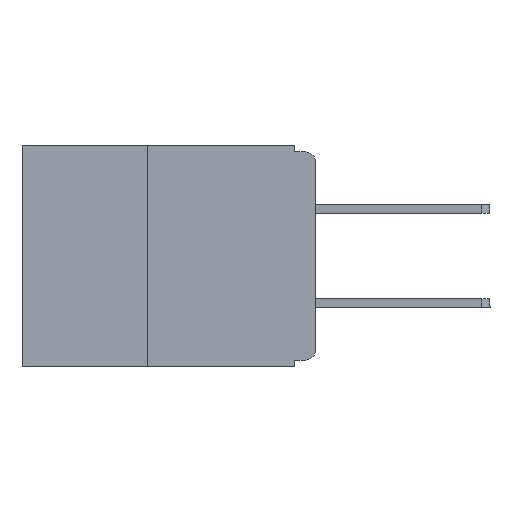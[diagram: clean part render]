
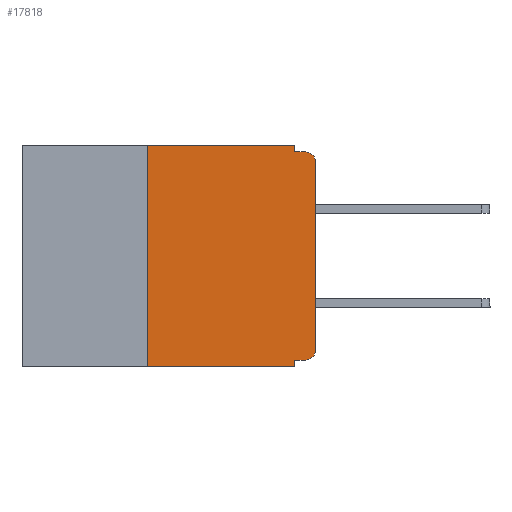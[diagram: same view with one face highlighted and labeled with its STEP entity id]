
A CAD part, left-side view. The second image highlights one B-rep face of the part: STEP entity #17818.
In plain terms, the highlighted planar face has unit normal (-1, 0, 0).
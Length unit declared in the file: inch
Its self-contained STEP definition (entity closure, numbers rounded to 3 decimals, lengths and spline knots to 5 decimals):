
#8 = CARTESIAN_POINT ( 'NONE',  ( 0., 0., 0. ) ) ;
#194 = CARTESIAN_POINT ( 'NONE',  ( 0., 0.25, 0. ) ) ;
#437 = LINE ( 'NONE', #5873, #7872 ) ;
#478 = DIRECTION ( 'NONE',  ( 0., 0., -1. ) ) ;
#487 = EDGE_CURVE ( 'NONE', #11605, #11095, #6424, .T. ) ;
#613 = ORIENTED_EDGE ( 'NONE', *, *, #2300, .F. ) ;
#980 = ORIENTED_EDGE ( 'NONE', *, *, #11216, .F. ) ;
#1407 = VERTEX_POINT ( 'NONE', #10038 ) ;
#1520 = DIRECTION ( 'NONE',  ( 0., 0., -1. ) ) ;
#1731 = LINE ( 'NONE', #17269, #12561 ) ;
#2257 = VECTOR ( 'NONE', #6563, 39.37008 ) ;
#2291 = AXIS2_PLACEMENT_3D ( 'NONE', #16004, #10372, #1520 ) ;
#2300 = EDGE_CURVE ( 'NONE', #6017, #14107, #12139, .T. ) ;
#2339 = ORIENTED_EDGE ( 'NONE', *, *, #15808, .F. ) ;
#2423 = VECTOR ( 'NONE', #478, 39.37008 ) ;
#2512 = CARTESIAN_POINT ( 'NONE',  ( 0., 0.015, -0.32 ) ) ;
#2629 = CARTESIAN_POINT ( 'NONE',  ( 0., 0.437, -0.33 ) ) ;
#2666 = EDGE_CURVE ( 'NONE', #6945, #1407, #1731, .T. ) ;
#2817 = VERTEX_POINT ( 'NONE', #13098 ) ;
#2829 = DIRECTION ( 'NONE',  ( 0., 0., -1. ) ) ;
#2949 = ORIENTED_EDGE ( 'NONE', *, *, #8596, .T. ) ;
#3160 = CARTESIAN_POINT ( 'NONE',  ( 0., 0.031, -0.33 ) ) ;
#3184 = EDGE_CURVE ( 'NONE', #6945, #11605, #4705, .T. ) ;
#3219 = LINE ( 'NONE', #2629, #10596 ) ;
#3246 = CARTESIAN_POINT ( 'NONE',  ( 0., 0.015, -0.025 ) ) ;
#3524 = VERTEX_POINT ( 'NONE', #194 ) ;
#4104 = DIRECTION ( 'NONE',  ( 0., -1., 0. ) ) ;
#4276 = EDGE_CURVE ( 'NONE', #3524, #2817, #437, .T. ) ;
#4498 = ORIENTED_EDGE ( 'NONE', *, *, #487, .T. ) ;
#4705 = CIRCLE ( 'NONE', #18412, 0.015 ) ;
#4715 = DIRECTION ( 'NONE',  ( 0., 0., -1. ) ) ;
#5078 = CARTESIAN_POINT ( 'NONE',  ( 0., 0.25, -0.33 ) ) ;
#5379 = ORIENTED_EDGE ( 'NONE', *, *, #3184, .T. ) ;
#5850 = DIRECTION ( 'NONE',  ( 0., -1., 0. ) ) ;
#5873 = CARTESIAN_POINT ( 'NONE',  ( 0., 0.437, 0. ) ) ;
#6017 = VERTEX_POINT ( 'NONE', #13529 ) ;
#6424 = LINE ( 'NONE', #8, #17345 ) ;
#6521 = FACE_OUTER_BOUND ( 'NONE', #8754, .T. ) ;
#6563 = DIRECTION ( 'NONE',  ( 0., 0., 1. ) ) ;
#6603 = VERTEX_POINT ( 'NONE', #3160 ) ;
#6945 = VERTEX_POINT ( 'NONE', #2512 ) ;
#7561 = CARTESIAN_POINT ( 'NONE',  ( 0., 0., -0.025 ) ) ;
#7872 = VECTOR ( 'NONE', #5850, 39.37008 ) ;
#8501 = ORIENTED_EDGE ( 'NONE', *, *, #14318, .F. ) ;
#8596 = EDGE_CURVE ( 'NONE', #11583, #6603, #3219, .T. ) ;
#8754 = EDGE_LOOP ( 'NONE', ( #4498, #16164, #613, #980, #10510, #2339, #2949, #8501, #18348, #5379 ) ) ;
#8821 = CARTESIAN_POINT ( 'NONE',  ( 0., 0., -0.305 ) ) ;
#8910 = EDGE_CURVE ( 'NONE', #11095, #14107, #16938, .T. ) ;
#9555 = CARTESIAN_POINT ( 'NONE',  ( 0., 0.015, -0.01 ) ) ;
#9629 = VECTOR ( 'NONE', #2829, 39.37008 ) ;
#10038 = CARTESIAN_POINT ( 'NONE',  ( 0., 0.031, -0.32 ) ) ;
#10268 = CARTESIAN_POINT ( 'NONE',  ( 0., 0.25, -0.33 ) ) ;
#10372 = DIRECTION ( 'NONE',  ( 1., 0., 0. ) ) ;
#10510 = ORIENTED_EDGE ( 'NONE', *, *, #4276, .F. ) ;
#10596 = VECTOR ( 'NONE', #4104, 39.37008 ) ;
#11095 = VERTEX_POINT ( 'NONE', #7561 ) ;
#11216 = EDGE_CURVE ( 'NONE', #2817, #6017, #14070, .T. ) ;
#11583 = VERTEX_POINT ( 'NONE', #10268 ) ;
#11605 = VERTEX_POINT ( 'NONE', #8821 ) ;
#11612 = AXIS2_PLACEMENT_3D ( 'NONE', #3246, #13475, #4715 ) ;
#11639 = DIRECTION ( 'NONE',  ( 0., 0., -1. ) ) ;
#11665 = CARTESIAN_POINT ( 'NONE',  ( 0., 0.031, -0.33 ) ) ;
#11726 = CARTESIAN_POINT ( 'NONE',  ( 0., 0.015, -0.305 ) ) ;
#11880 = DIRECTION ( 'NONE',  ( 0., -1., 0. ) ) ;
#11913 = DIRECTION ( 'NONE',  ( -1., 0., 0. ) ) ;
#12139 = LINE ( 'NONE', #13084, #16666 ) ;
#12561 = VECTOR ( 'NONE', #14027, 39.37008 ) ;
#13034 = LINE ( 'NONE', #5078, #2257 ) ;
#13084 = CARTESIAN_POINT ( 'NONE',  ( 0., 0., -0.01 ) ) ;
#13098 = CARTESIAN_POINT ( 'NONE',  ( 0., 0.031, 0. ) ) ;
#13475 = DIRECTION ( 'NONE',  ( -1., 0., 0. ) ) ;
#13529 = CARTESIAN_POINT ( 'NONE',  ( 0., 0.031, -0.01 ) ) ;
#14027 = DIRECTION ( 'NONE',  ( 0., 1., 0. ) ) ;
#14070 = LINE ( 'NONE', #17769, #2423 ) ;
#14107 = VERTEX_POINT ( 'NONE', #9555 ) ;
#14318 = EDGE_CURVE ( 'NONE', #1407, #6603, #16294, .T. ) ;
#14752 = DIRECTION ( 'NONE',  ( 0., 0., 1. ) ) ;
#15808 = EDGE_CURVE ( 'NONE', #11583, #3524, #13034, .T. ) ;
#16004 = CARTESIAN_POINT ( 'NONE',  ( 0., 0.437, 0. ) ) ;
#16164 = ORIENTED_EDGE ( 'NONE', *, *, #8910, .T. ) ;
#16294 = LINE ( 'NONE', #11665, #9629 ) ;
#16666 = VECTOR ( 'NONE', #11880, 39.37008 ) ;
#16938 = CIRCLE ( 'NONE', #11612, 0.015 ) ;
#17269 = CARTESIAN_POINT ( 'NONE',  ( 0., 0., -0.32 ) ) ;
#17345 = VECTOR ( 'NONE', #14752, 39.37008 ) ;
#17769 = CARTESIAN_POINT ( 'NONE',  ( 0., 0.031, 0. ) ) ;
#17818 = ADVANCED_FACE ( 'NONE', ( #6521 ), #18645, .F. ) ;
#18348 = ORIENTED_EDGE ( 'NONE', *, *, #2666, .F. ) ;
#18412 = AXIS2_PLACEMENT_3D ( 'NONE', #11726, #11913, #11639 ) ;
#18645 = PLANE ( 'NONE',  #2291 ) ;
